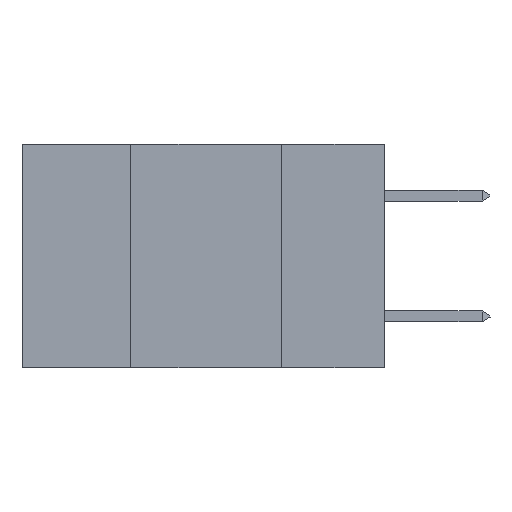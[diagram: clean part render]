
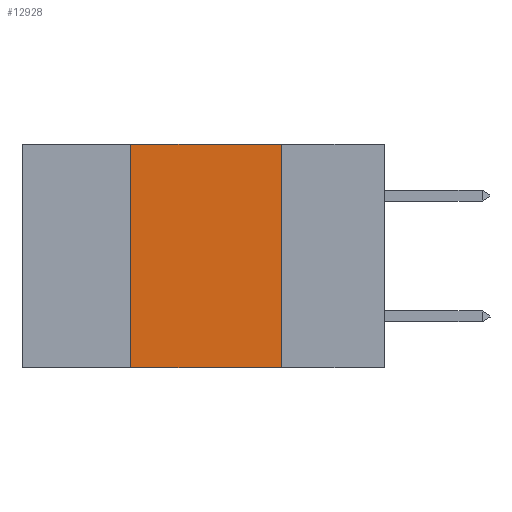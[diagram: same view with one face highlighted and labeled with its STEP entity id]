
A CAD part, left-side view. The second image highlights one B-rep face of the part: STEP entity #12928.
In plain terms, the highlighted planar face has unit normal (-1, 0, 0).
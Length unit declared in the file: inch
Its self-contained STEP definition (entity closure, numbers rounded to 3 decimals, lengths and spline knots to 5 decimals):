
#536 = ORIENTED_EDGE ( 'NONE', *, *, #5282, .F. ) ;
#1049 = CARTESIAN_POINT ( 'NONE',  ( 0., 0.17, -0.37 ) ) ;
#2178 = VERTEX_POINT ( 'NONE', #16288 ) ;
#2245 = DIRECTION ( 'NONE',  ( 0., 0., -1. ) ) ;
#2477 = DIRECTION ( 'NONE',  ( 1., 0., 0. ) ) ;
#2706 = ORIENTED_EDGE ( 'NONE', *, *, #16687, .F. ) ;
#2727 = AXIS2_PLACEMENT_3D ( 'NONE', #8697, #2477, #13522 ) ;
#2990 = CARTESIAN_POINT ( 'NONE',  ( 0., 0.17, 0. ) ) ;
#3541 = LINE ( 'NONE', #11669, #15670 ) ;
#4754 = VECTOR ( 'NONE', #11134, 39.37008 ) ;
#4923 = EDGE_CURVE ( 'NONE', #5533, #18946, #14216, .T. ) ;
#5282 = EDGE_CURVE ( 'NONE', #15221, #18946, #3541, .T. ) ;
#5533 = VERTEX_POINT ( 'NONE', #16974 ) ;
#5729 = VECTOR ( 'NONE', #9228, 39.37008 ) ;
#7114 = ORIENTED_EDGE ( 'NONE', *, *, #19372, .F. ) ;
#7649 = CARTESIAN_POINT ( 'NONE',  ( 0., 0.6, -0.37 ) ) ;
#8079 = VECTOR ( 'NONE', #11475, 39.37008 ) ;
#8697 = CARTESIAN_POINT ( 'NONE',  ( 0., 0.6, 0. ) ) ;
#9228 = DIRECTION ( 'NONE',  ( 0., -1., 0. ) ) ;
#9847 = CARTESIAN_POINT ( 'NONE',  ( 0., 0.6, 0. ) ) ;
#10507 = EDGE_LOOP ( 'NONE', ( #536, #7114, #2706, #11559 ) ) ;
#11134 = DIRECTION ( 'NONE',  ( 0., 0., 1. ) ) ;
#11475 = DIRECTION ( 'NONE',  ( 0., -1., 0. ) ) ;
#11559 = ORIENTED_EDGE ( 'NONE', *, *, #4923, .T. ) ;
#11669 = CARTESIAN_POINT ( 'NONE',  ( 0., 0.17, 0. ) ) ;
#12928 = ADVANCED_FACE ( 'NONE', ( #16335 ), #19677, .F. ) ;
#13522 = DIRECTION ( 'NONE',  ( 0., 0., -1. ) ) ;
#14216 = LINE ( 'NONE', #7649, #5729 ) ;
#15221 = VERTEX_POINT ( 'NONE', #2990 ) ;
#15670 = VECTOR ( 'NONE', #2245, 39.37008 ) ;
#16288 = CARTESIAN_POINT ( 'NONE',  ( 0., 0.42, 0. ) ) ;
#16335 = FACE_OUTER_BOUND ( 'NONE', #10507, .T. ) ;
#16510 = LINE ( 'NONE', #9847, #8079 ) ;
#16687 = EDGE_CURVE ( 'NONE', #5533, #2178, #17381, .T. ) ;
#16974 = CARTESIAN_POINT ( 'NONE',  ( 0., 0.42, -0.37 ) ) ;
#17381 = LINE ( 'NONE', #19014, #4754 ) ;
#18946 = VERTEX_POINT ( 'NONE', #1049 ) ;
#19014 = CARTESIAN_POINT ( 'NONE',  ( 0., 0.42, 0. ) ) ;
#19372 = EDGE_CURVE ( 'NONE', #2178, #15221, #16510, .T. ) ;
#19677 = PLANE ( 'NONE',  #2727 ) ;
